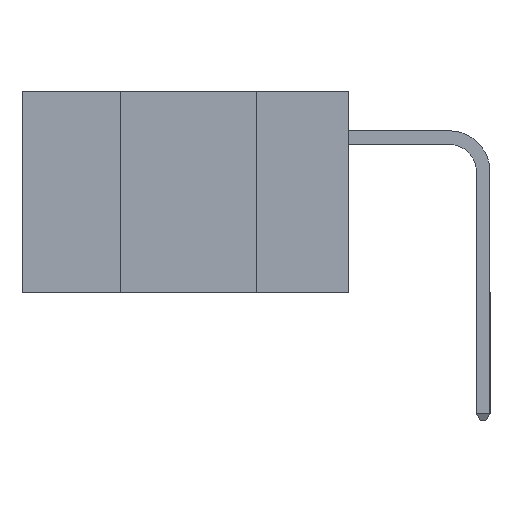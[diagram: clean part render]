
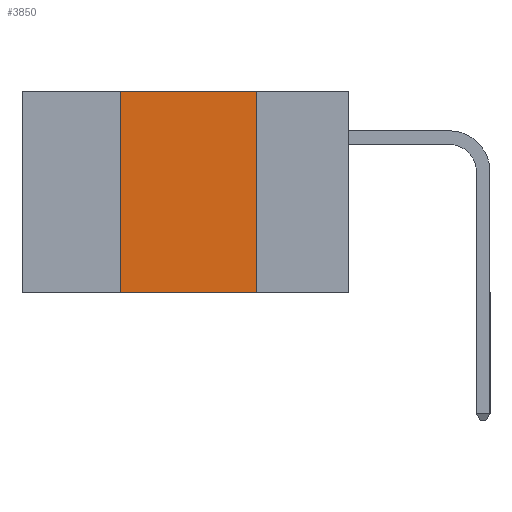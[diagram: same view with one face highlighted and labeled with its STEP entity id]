
A CAD part, left-side view. The second image highlights one B-rep face of the part: STEP entity #3850.
In plain terms, the highlighted planar face has unit normal (-1, 0, 0).
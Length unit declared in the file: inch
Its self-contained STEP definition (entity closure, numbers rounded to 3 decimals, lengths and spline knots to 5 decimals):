
#574 = EDGE_CURVE ( 'NONE', #6108, #7488, #5735, .T. ) ;
#1145 = ORIENTED_EDGE ( 'NONE', *, *, #9672, .F. ) ;
#1706 = CARTESIAN_POINT ( 'NONE',  ( 0., 0.6, -0.37 ) ) ;
#1844 = ORIENTED_EDGE ( 'NONE', *, *, #574, .F. ) ;
#2056 = CARTESIAN_POINT ( 'NONE',  ( 0., 0.6, 0. ) ) ;
#2461 = VERTEX_POINT ( 'NONE', #10836 ) ;
#2472 = CARTESIAN_POINT ( 'NONE',  ( 0., 0.17, 0. ) ) ;
#2702 = ORIENTED_EDGE ( 'NONE', *, *, #9432, .F. ) ;
#3273 = LINE ( 'NONE', #7916, #7288 ) ;
#3728 = ORIENTED_EDGE ( 'NONE', *, *, #6339, .T. ) ;
#3850 = ADVANCED_FACE ( 'NONE', ( #6923 ), #10594, .F. ) ;
#4634 = DIRECTION ( 'NONE',  ( 1., 0., 0. ) ) ;
#4771 = DIRECTION ( 'NONE',  ( 0., 0., -1. ) ) ;
#4838 = DIRECTION ( 'NONE',  ( 0., -1., 0. ) ) ;
#5480 = VECTOR ( 'NONE', #9896, 39.37008 ) ;
#5613 = VECTOR ( 'NONE', #5876, 39.37008 ) ;
#5735 = LINE ( 'NONE', #7651, #5480 ) ;
#5876 = DIRECTION ( 'NONE',  ( 0., 0., -1. ) ) ;
#6065 = CARTESIAN_POINT ( 'NONE',  ( 0., 0.17, -0.37 ) ) ;
#6108 = VERTEX_POINT ( 'NONE', #8549 ) ;
#6339 = EDGE_CURVE ( 'NONE', #6108, #9870, #9100, .T. ) ;
#6876 = VECTOR ( 'NONE', #8094, 39.37008 ) ;
#6923 = FACE_OUTER_BOUND ( 'NONE', #9443, .T. ) ;
#7288 = VECTOR ( 'NONE', #4838, 39.37008 ) ;
#7488 = VERTEX_POINT ( 'NONE', #10425 ) ;
#7630 = LINE ( 'NONE', #2472, #5613 ) ;
#7651 = CARTESIAN_POINT ( 'NONE',  ( 0., 0.42, 0. ) ) ;
#7916 = CARTESIAN_POINT ( 'NONE',  ( 0., 0.6, 0. ) ) ;
#8094 = DIRECTION ( 'NONE',  ( 0., -1., 0. ) ) ;
#8549 = CARTESIAN_POINT ( 'NONE',  ( 0., 0.42, -0.37 ) ) ;
#9100 = LINE ( 'NONE', #1706, #6876 ) ;
#9432 = EDGE_CURVE ( 'NONE', #7488, #2461, #3273, .T. ) ;
#9443 = EDGE_LOOP ( 'NONE', ( #1145, #2702, #1844, #3728 ) ) ;
#9672 = EDGE_CURVE ( 'NONE', #2461, #9870, #7630, .T. ) ;
#9870 = VERTEX_POINT ( 'NONE', #6065 ) ;
#9896 = DIRECTION ( 'NONE',  ( 0., 0., 1. ) ) ;
#10425 = CARTESIAN_POINT ( 'NONE',  ( 0., 0.42, 0. ) ) ;
#10594 = PLANE ( 'NONE',  #10726 ) ;
#10726 = AXIS2_PLACEMENT_3D ( 'NONE', #2056, #4634, #4771 ) ;
#10836 = CARTESIAN_POINT ( 'NONE',  ( 0., 0.17, 0. ) ) ;
